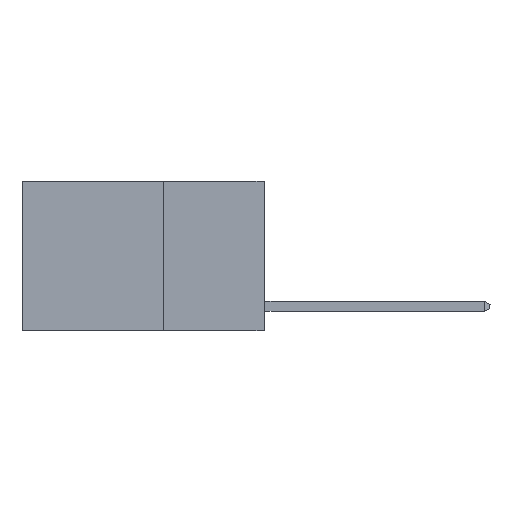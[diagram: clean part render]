
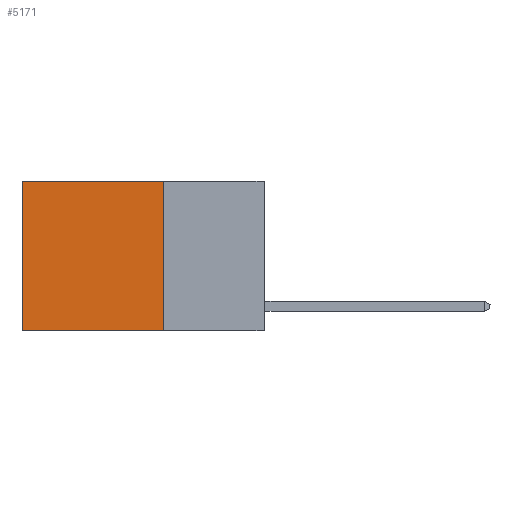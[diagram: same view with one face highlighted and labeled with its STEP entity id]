
A CAD part, left-side view. The second image highlights one B-rep face of the part: STEP entity #5171.
In plain terms, the highlighted planar face has unit normal (-1, 0, 0).
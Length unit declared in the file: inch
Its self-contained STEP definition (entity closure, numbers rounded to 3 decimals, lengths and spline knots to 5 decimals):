
#1316 = DIRECTION ( 'NONE',  ( 0., 0., -1. ) ) ;
#1512 = EDGE_CURVE ( 'NONE', #3760, #6086, #5633, .T. ) ;
#1574 = CARTESIAN_POINT ( 'NONE',  ( 0.2625, 0.6, 0. ) ) ;
#1578 = ORIENTED_EDGE ( 'NONE', *, *, #7458, .F. ) ;
#1675 = DIRECTION ( 'NONE',  ( 0., 0., -1. ) ) ;
#2231 = EDGE_CURVE ( 'NONE', #8443, #3760, #8008, .T. ) ;
#2619 = FACE_OUTER_BOUND ( 'NONE', #12306, .T. ) ;
#2755 = CARTESIAN_POINT ( 'NONE',  ( 0.2625, 0.25, 0. ) ) ;
#3104 = CARTESIAN_POINT ( 'NONE',  ( 0.2625, 0.25, 0. ) ) ;
#3121 = CARTESIAN_POINT ( 'NONE',  ( 0.2625, 0.25, -0.37 ) ) ;
#3365 = ORIENTED_EDGE ( 'NONE', *, *, #1512, .T. ) ;
#3370 = ORIENTED_EDGE ( 'NONE', *, *, #5935, .F. ) ;
#3760 = VERTEX_POINT ( 'NONE', #1574 ) ;
#3898 = ORIENTED_EDGE ( 'NONE', *, *, #2231, .T. ) ;
#4144 = VECTOR ( 'NONE', #4800, 39.37008 ) ;
#4768 = VECTOR ( 'NONE', #1316, 39.37008 ) ;
#4800 = DIRECTION ( 'NONE',  ( 0., 0., -1. ) ) ;
#5171 = ADVANCED_FACE ( 'NONE', ( #2619 ), #11219, .F. ) ;
#5525 = CARTESIAN_POINT ( 'NONE',  ( 0.2625, 0.25, 0. ) ) ;
#5633 = LINE ( 'NONE', #7660, #4144 ) ;
#5935 = EDGE_CURVE ( 'NONE', #8443, #7284, #12410, .T. ) ;
#6086 = VERTEX_POINT ( 'NONE', #9297 ) ;
#7284 = VERTEX_POINT ( 'NONE', #8495 ) ;
#7458 = EDGE_CURVE ( 'NONE', #7284, #6086, #11880, .T. ) ;
#7499 = DIRECTION ( 'NONE',  ( 1., 0., 0. ) ) ;
#7660 = CARTESIAN_POINT ( 'NONE',  ( 0.2625, 0.6, 0. ) ) ;
#8008 = LINE ( 'NONE', #9481, #10979 ) ;
#8443 = VERTEX_POINT ( 'NONE', #2755 ) ;
#8449 = DIRECTION ( 'NONE',  ( 0., 1., 0. ) ) ;
#8495 = CARTESIAN_POINT ( 'NONE',  ( 0.2625, 0.25, -0.37 ) ) ;
#8741 = VECTOR ( 'NONE', #8905, 39.37008 ) ;
#8905 = DIRECTION ( 'NONE',  ( 0., 1., 0. ) ) ;
#9297 = CARTESIAN_POINT ( 'NONE',  ( 0.2625, 0.6, -0.37 ) ) ;
#9481 = CARTESIAN_POINT ( 'NONE',  ( 0.2625, 0.25, 0. ) ) ;
#10439 = AXIS2_PLACEMENT_3D ( 'NONE', #5525, #7499, #1675 ) ;
#10979 = VECTOR ( 'NONE', #8449, 39.37008 ) ;
#11219 = PLANE ( 'NONE',  #10439 ) ;
#11880 = LINE ( 'NONE', #3121, #8741 ) ;
#12306 = EDGE_LOOP ( 'NONE', ( #3365, #1578, #3370, #3898 ) ) ;
#12410 = LINE ( 'NONE', #3104, #4768 ) ;
